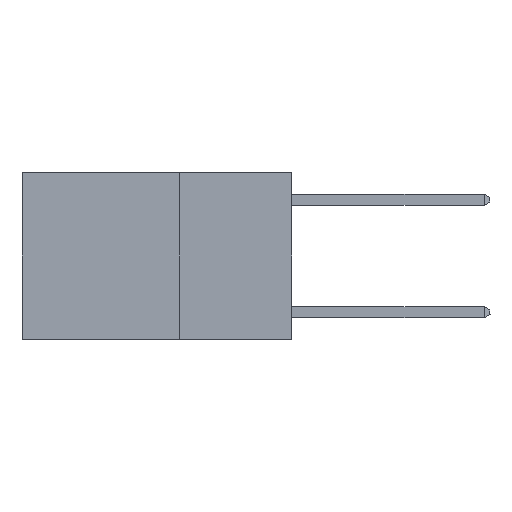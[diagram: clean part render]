
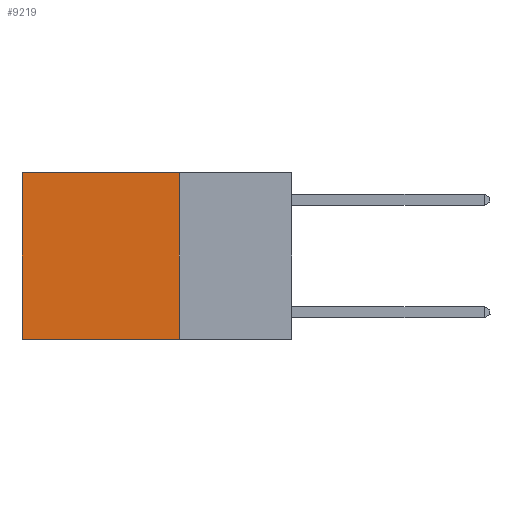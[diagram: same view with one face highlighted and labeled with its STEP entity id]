
A CAD part, left-side view. The second image highlights one B-rep face of the part: STEP entity #9219.
In plain terms, the highlighted planar face has unit normal (-1, 0, 0).
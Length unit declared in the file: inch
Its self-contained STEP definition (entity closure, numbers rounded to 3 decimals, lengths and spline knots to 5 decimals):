
#7 = CARTESIAN_POINT ( 'NONE',  ( 0.2625, 0.25, 0. ) ) ;
#290 = CARTESIAN_POINT ( 'NONE',  ( 0.2625, 0.25, 0. ) ) ;
#332 = AXIS2_PLACEMENT_3D ( 'NONE', #290, #2836, #5376 ) ;
#730 = LINE ( 'NONE', #7411, #10548 ) ;
#1335 = VERTEX_POINT ( 'NONE', #7009 ) ;
#1919 = EDGE_CURVE ( 'NONE', #4819, #6418, #8860, .T. ) ;
#2614 = ORIENTED_EDGE ( 'NONE', *, *, #8932, .F. ) ;
#2656 = EDGE_LOOP ( 'NONE', ( #5354, #9145, #2614, #2986 ) ) ;
#2836 = DIRECTION ( 'NONE',  ( 1., 0., 0. ) ) ;
#2986 = ORIENTED_EDGE ( 'NONE', *, *, #6060, .T. ) ;
#3252 = DIRECTION ( 'NONE',  ( 0., 1., 0. ) ) ;
#3262 = VECTOR ( 'NONE', #8954, 39.37008 ) ;
#4025 = CARTESIAN_POINT ( 'NONE',  ( 0.2625, 0.25, 0. ) ) ;
#4042 = LINE ( 'NONE', #4802, #3262 ) ;
#4802 = CARTESIAN_POINT ( 'NONE',  ( 0.2625, 0.25, -0.37 ) ) ;
#4819 = VERTEX_POINT ( 'NONE', #7457 ) ;
#5321 = VERTEX_POINT ( 'NONE', #4025 ) ;
#5322 = FACE_OUTER_BOUND ( 'NONE', #2656, .T. ) ;
#5354 = ORIENTED_EDGE ( 'NONE', *, *, #1919, .T. ) ;
#5376 = DIRECTION ( 'NONE',  ( 0., 0., -1. ) ) ;
#6029 = LINE ( 'NONE', #7, #9187 ) ;
#6060 = EDGE_CURVE ( 'NONE', #5321, #4819, #730, .T. ) ;
#6418 = VERTEX_POINT ( 'NONE', #7347 ) ;
#6619 = DIRECTION ( 'NONE',  ( 0., 0., -1. ) ) ;
#7009 = CARTESIAN_POINT ( 'NONE',  ( 0.2625, 0.25, -0.37 ) ) ;
#7046 = CARTESIAN_POINT ( 'NONE',  ( 0.2625, 0.6, 0. ) ) ;
#7208 = DIRECTION ( 'NONE',  ( 0., 0., -1. ) ) ;
#7347 = CARTESIAN_POINT ( 'NONE',  ( 0.2625, 0.6, -0.37 ) ) ;
#7411 = CARTESIAN_POINT ( 'NONE',  ( 0.2625, 0.25, 0. ) ) ;
#7457 = CARTESIAN_POINT ( 'NONE',  ( 0.2625, 0.6, 0. ) ) ;
#7774 = EDGE_CURVE ( 'NONE', #1335, #6418, #4042, .T. ) ;
#7817 = VECTOR ( 'NONE', #7208, 39.37008 ) ;
#8703 = PLANE ( 'NONE',  #332 ) ;
#8860 = LINE ( 'NONE', #7046, #7817 ) ;
#8932 = EDGE_CURVE ( 'NONE', #5321, #1335, #6029, .T. ) ;
#8954 = DIRECTION ( 'NONE',  ( 0., 1., 0. ) ) ;
#9145 = ORIENTED_EDGE ( 'NONE', *, *, #7774, .F. ) ;
#9187 = VECTOR ( 'NONE', #6619, 39.37008 ) ;
#9219 = ADVANCED_FACE ( 'NONE', ( #5322 ), #8703, .F. ) ;
#10548 = VECTOR ( 'NONE', #3252, 39.37008 ) ;
